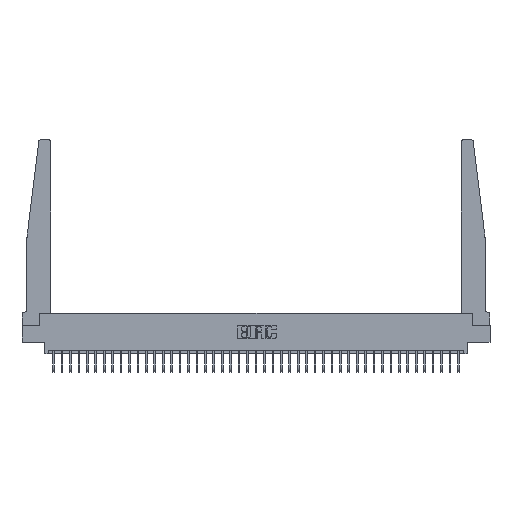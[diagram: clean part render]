
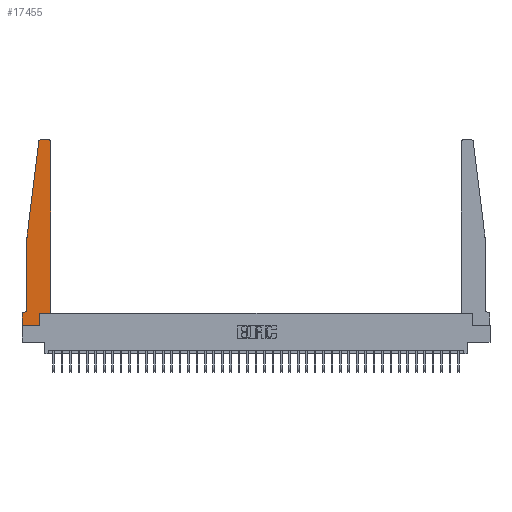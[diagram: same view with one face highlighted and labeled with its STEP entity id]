
A CAD part, top view. The second image highlights one B-rep face of the part: STEP entity #17455.
In plain terms, the highlighted planar face has unit normal (0, 0, 1).
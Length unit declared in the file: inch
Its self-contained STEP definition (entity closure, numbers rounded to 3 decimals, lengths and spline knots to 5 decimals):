
#127 = AXIS2_PLACEMENT_3D ( 'NONE', #11739, #5859, #29503 ) ;
#157 = VERTEX_POINT ( 'NONE', #16990 ) ;
#978 = VECTOR ( 'NONE', #7320, 39.37008 ) ;
#1111 = CARTESIAN_POINT ( 'NONE',  ( 0., 0., 0.37 ) ) ;
#1164 = DIRECTION ( 'NONE',  ( -1., 0., 0. ) ) ;
#1222 = VECTOR ( 'NONE', #26270, 39.37008 ) ;
#1451 = DIRECTION ( 'NONE',  ( 0., 0., 1. ) ) ;
#1485 = DIRECTION ( 'NONE',  ( 0., -1., 0. ) ) ;
#1973 = CARTESIAN_POINT ( 'NONE',  ( 0.065, 1.25, 0.37 ) ) ;
#2036 = EDGE_CURVE ( 'NONE', #16141, #157, #33979, .T. ) ;
#2556 = CARTESIAN_POINT ( 'NONE',  ( 0.015, 0.1875, 0.37 ) ) ;
#3641 = CIRCLE ( 'NONE', #127, 0.03 ) ;
#4712 = VECTOR ( 'NONE', #33823, 39.37008 ) ;
#5184 = LINE ( 'NONE', #12950, #978 ) ;
#5338 = CARTESIAN_POINT ( 'NONE',  ( 0., 0., 0.37 ) ) ;
#5453 = VERTEX_POINT ( 'NONE', #23559 ) ;
#5859 = DIRECTION ( 'NONE',  ( 0., 0., 1. ) ) ;
#5962 = CARTESIAN_POINT ( 'NONE',  ( 0.395, 2.75, 0.37 ) ) ;
#6072 = VERTEX_POINT ( 'NONE', #5962 ) ;
#6552 = EDGE_CURVE ( 'NONE', #37663, #35189, #14503, .T. ) ;
#6889 = DIRECTION ( 'NONE',  ( 0., 0., -1. ) ) ;
#7320 = DIRECTION ( 'NONE',  ( -1., 0., 0. ) ) ;
#7387 = ORIENTED_EDGE ( 'NONE', *, *, #21715, .T. ) ;
#7723 = DIRECTION ( 'NONE',  ( 0., -1., 0. ) ) ;
#8037 = VERTEX_POINT ( 'NONE', #16124 ) ;
#8816 = ORIENTED_EDGE ( 'NONE', *, *, #11403, .T. ) ;
#11103 = CARTESIAN_POINT ( 'NONE',  ( 0.2605, 0.18, 0.37 ) ) ;
#11382 = EDGE_CURVE ( 'NONE', #32111, #8037, #29207, .T. ) ;
#11403 = EDGE_CURVE ( 'NONE', #19151, #24334, #25485, .T. ) ;
#11739 = CARTESIAN_POINT ( 'NONE',  ( 0.395, 2.72, 0.37 ) ) ;
#12516 = FACE_OUTER_BOUND ( 'NONE', #13718, .T. ) ;
#12950 = CARTESIAN_POINT ( 'NONE',  ( 0.25, 2.75, 0.37 ) ) ;
#12951 = DIRECTION ( 'NONE',  ( 1., 0., 0. ) ) ;
#13718 = EDGE_LOOP ( 'NONE', ( #28732, #29104, #23957, #22162, #8816, #7387, #35997, #15172, #26667, #28615, #31241, #30381 ) ) ;
#13926 = AXIS2_PLACEMENT_3D ( 'NONE', #18660, #6889, #1164 ) ;
#14437 = DIRECTION ( 'NONE',  ( 1., 0., 0. ) ) ;
#14442 = EDGE_CURVE ( 'NONE', #6072, #30338, #5184, .T. ) ;
#14503 = LINE ( 'NONE', #1111, #34999 ) ;
#14942 = VERTEX_POINT ( 'NONE', #26710 ) ;
#14950 = LINE ( 'NONE', #25602, #27745 ) ;
#15172 = ORIENTED_EDGE ( 'NONE', *, *, #36128, .T. ) ;
#15213 = LINE ( 'NONE', #20148, #27562 ) ;
#15643 = CARTESIAN_POINT ( 'NONE',  ( 0.27653, 2.72, 0.37 ) ) ;
#16124 = CARTESIAN_POINT ( 'NONE',  ( 0.065, 1.25, 0.37 ) ) ;
#16141 = VERTEX_POINT ( 'NONE', #35600 ) ;
#16337 = LINE ( 'NONE', #1973, #28223 ) ;
#16890 = EDGE_CURVE ( 'NONE', #30338, #32111, #23943, .T. ) ;
#16990 = CARTESIAN_POINT ( 'NONE',  ( 0.425, 2.72, 0.37 ) ) ;
#17241 = CARTESIAN_POINT ( 'NONE',  ( 0.065, 0.1875, 0.37 ) ) ;
#17455 = ADVANCED_FACE ( 'NONE', ( #12516 ), #37171, .T. ) ;
#17919 = AXIS2_PLACEMENT_3D ( 'NONE', #15643, #1451, #12951 ) ;
#18431 = CARTESIAN_POINT ( 'NONE',  ( 0.065, 0.2375, 0.37 ) ) ;
#18660 = CARTESIAN_POINT ( 'NONE',  ( 0.015, 0.2375, 0.37 ) ) ;
#18678 = VECTOR ( 'NONE', #26831, 39.37008 ) ;
#19151 = VERTEX_POINT ( 'NONE', #18431 ) ;
#19990 = LINE ( 'NONE', #11103, #36792 ) ;
#20148 = CARTESIAN_POINT ( 'NONE',  ( 0.425, 0.18, 0.37 ) ) ;
#21478 = EDGE_CURVE ( 'NONE', #8037, #19151, #16337, .T. ) ;
#21715 = EDGE_CURVE ( 'NONE', #24334, #37663, #25422, .T. ) ;
#22015 = EDGE_CURVE ( 'NONE', #5453, #14942, #19990, .T. ) ;
#22162 = ORIENTED_EDGE ( 'NONE', *, *, #21478, .T. ) ;
#22507 = DIRECTION ( 'NONE',  ( 1., 0., 0. ) ) ;
#22824 = DIRECTION ( 'NONE',  ( 0., 1., 0. ) ) ;
#23559 = CARTESIAN_POINT ( 'NONE',  ( 0.2605, 0., 0.37 ) ) ;
#23943 = CIRCLE ( 'NONE', #17919, 0.03 ) ;
#23957 = ORIENTED_EDGE ( 'NONE', *, *, #11382, .T. ) ;
#24334 = VERTEX_POINT ( 'NONE', #2556 ) ;
#24719 = CARTESIAN_POINT ( 'NONE',  ( 0.425, 0.18, 0.37 ) ) ;
#25422 = LINE ( 'NONE', #17241, #1222 ) ;
#25485 = CIRCLE ( 'NONE', #13926, 0.05 ) ;
#25602 = CARTESIAN_POINT ( 'NONE',  ( 0., 0., 0.37 ) ) ;
#26261 = CARTESIAN_POINT ( 'NONE',  ( 0.27653, 2.75, 0.37 ) ) ;
#26270 = DIRECTION ( 'NONE',  ( -1., 0., 0. ) ) ;
#26667 = ORIENTED_EDGE ( 'NONE', *, *, #22015, .T. ) ;
#26710 = CARTESIAN_POINT ( 'NONE',  ( 0.2605, 0.18, 0.37 ) ) ;
#26831 = DIRECTION ( 'NONE',  ( -0.122, -0.992, 0. ) ) ;
#27474 = DIRECTION ( 'NONE',  ( 0., 0., 1. ) ) ;
#27562 = VECTOR ( 'NONE', #14437, 39.37008 ) ;
#27745 = VECTOR ( 'NONE', #22507, 39.37008 ) ;
#28223 = VECTOR ( 'NONE', #7723, 39.37008 ) ;
#28615 = ORIENTED_EDGE ( 'NONE', *, *, #34051, .T. ) ;
#28732 = ORIENTED_EDGE ( 'NONE', *, *, #14442, .T. ) ;
#29104 = ORIENTED_EDGE ( 'NONE', *, *, #16890, .T. ) ;
#29207 = LINE ( 'NONE', #32586, #18678 ) ;
#29503 = DIRECTION ( 'NONE',  ( 1., 0., 0. ) ) ;
#29720 = EDGE_CURVE ( 'NONE', #157, #6072, #3641, .T. ) ;
#30265 = DIRECTION ( 'NONE',  ( 1., 0., 0. ) ) ;
#30338 = VERTEX_POINT ( 'NONE', #26261 ) ;
#30381 = ORIENTED_EDGE ( 'NONE', *, *, #29720, .T. ) ;
#31241 = ORIENTED_EDGE ( 'NONE', *, *, #2036, .T. ) ;
#32111 = VERTEX_POINT ( 'NONE', #37199 ) ;
#32586 = CARTESIAN_POINT ( 'NONE',  ( 0.065, 1.25, 0.37 ) ) ;
#33823 = DIRECTION ( 'NONE',  ( 0., 1., 0. ) ) ;
#33979 = LINE ( 'NONE', #24719, #4712 ) ;
#34051 = EDGE_CURVE ( 'NONE', #14942, #16141, #15213, .T. ) ;
#34791 = AXIS2_PLACEMENT_3D ( 'NONE', #35730, #27474, #30265 ) ;
#34999 = VECTOR ( 'NONE', #1485, 39.37008 ) ;
#35189 = VERTEX_POINT ( 'NONE', #5338 ) ;
#35600 = CARTESIAN_POINT ( 'NONE',  ( 0.425, 0.18, 0.37 ) ) ;
#35730 = CARTESIAN_POINT ( 'NONE',  ( 0., 0.1875, 0.37 ) ) ;
#35790 = CARTESIAN_POINT ( 'NONE',  ( 0., 0.1875, 0.37 ) ) ;
#35997 = ORIENTED_EDGE ( 'NONE', *, *, #6552, .T. ) ;
#36128 = EDGE_CURVE ( 'NONE', #35189, #5453, #14950, .T. ) ;
#36792 = VECTOR ( 'NONE', #22824, 39.37008 ) ;
#37171 = PLANE ( 'NONE',  #34791 ) ;
#37199 = CARTESIAN_POINT ( 'NONE',  ( 0.24675, 2.72367, 0.37 ) ) ;
#37663 = VERTEX_POINT ( 'NONE', #35790 ) ;
